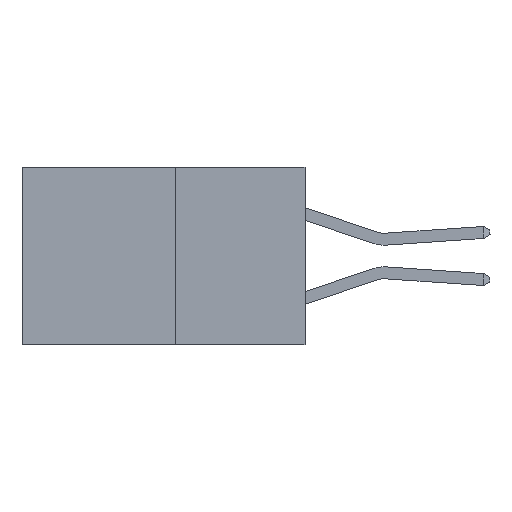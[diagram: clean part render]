
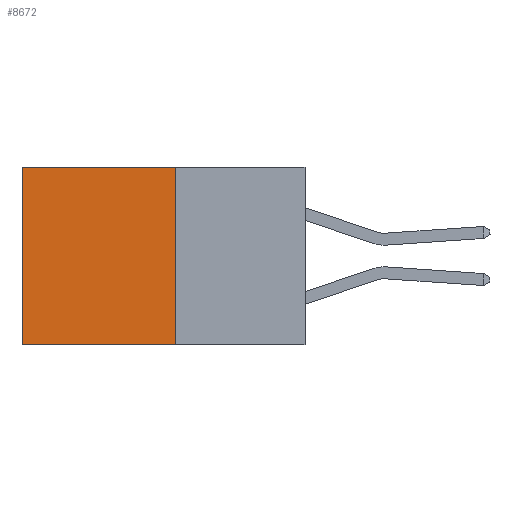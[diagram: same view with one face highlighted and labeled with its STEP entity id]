
A CAD part, left-side view. The second image highlights one B-rep face of the part: STEP entity #8672.
In plain terms, the highlighted planar face has unit normal (-1, 0, 0).
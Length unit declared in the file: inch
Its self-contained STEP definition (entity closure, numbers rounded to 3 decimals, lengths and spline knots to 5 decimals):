
#393 = EDGE_CURVE ( 'NONE', #8208, #5028, #4133, .T. ) ;
#781 = VECTOR ( 'NONE', #8328, 39.37008 ) ;
#1200 = VERTEX_POINT ( 'NONE', #11657 ) ;
#1939 = VERTEX_POINT ( 'NONE', #8195 ) ;
#2262 = CARTESIAN_POINT ( 'NONE',  ( 0.277, 0.59, -0.37 ) ) ;
#3747 = FACE_OUTER_BOUND ( 'NONE', #6007, .T. ) ;
#4133 = LINE ( 'NONE', #11971, #781 ) ;
#5028 = VERTEX_POINT ( 'NONE', #6715 ) ;
#5177 = EDGE_CURVE ( 'NONE', #1939, #1200, #8496, .T. ) ;
#5784 = VECTOR ( 'NONE', #11952, 39.37008 ) ;
#5949 = VECTOR ( 'NONE', #14698, 39.37008 ) ;
#6007 = EDGE_LOOP ( 'NONE', ( #10466, #9298, #6360, #11287 ) ) ;
#6179 = PLANE ( 'NONE',  #8177 ) ;
#6360 = ORIENTED_EDGE ( 'NONE', *, *, #15496, .F. ) ;
#6715 = CARTESIAN_POINT ( 'NONE',  ( 0.277, 0.59, 0. ) ) ;
#7384 = CARTESIAN_POINT ( 'NONE',  ( 0.277, 0.27, -0.37 ) ) ;
#8134 = VECTOR ( 'NONE', #11903, 39.37008 ) ;
#8177 = AXIS2_PLACEMENT_3D ( 'NONE', #7384, #15830, #8609 ) ;
#8195 = CARTESIAN_POINT ( 'NONE',  ( 0.277, 0.27, -0.37 ) ) ;
#8208 = VERTEX_POINT ( 'NONE', #11421 ) ;
#8328 = DIRECTION ( 'NONE',  ( 0., 1., 0. ) ) ;
#8496 = LINE ( 'NONE', #15437, #8134 ) ;
#8609 = DIRECTION ( 'NONE',  ( 0., 0., -1. ) ) ;
#8672 = ADVANCED_FACE ( 'NONE', ( #3747 ), #6179, .F. ) ;
#8994 = LINE ( 'NONE', #2262, #5784 ) ;
#9298 = ORIENTED_EDGE ( 'NONE', *, *, #5177, .F. ) ;
#10466 = ORIENTED_EDGE ( 'NONE', *, *, #15181, .T. ) ;
#11287 = ORIENTED_EDGE ( 'NONE', *, *, #393, .T. ) ;
#11421 = CARTESIAN_POINT ( 'NONE',  ( 0.277, 0.27, 0. ) ) ;
#11657 = CARTESIAN_POINT ( 'NONE',  ( 0.277, 0.59, -0.37 ) ) ;
#11903 = DIRECTION ( 'NONE',  ( 0., 1., 0. ) ) ;
#11952 = DIRECTION ( 'NONE',  ( 0., 0., -1. ) ) ;
#11971 = CARTESIAN_POINT ( 'NONE',  ( 0.277, 0.27, 0. ) ) ;
#12449 = LINE ( 'NONE', #13508, #5949 ) ;
#13508 = CARTESIAN_POINT ( 'NONE',  ( 0.277, 0.27, -0.37 ) ) ;
#14698 = DIRECTION ( 'NONE',  ( 0., 0., -1. ) ) ;
#15181 = EDGE_CURVE ( 'NONE', #5028, #1200, #8994, .T. ) ;
#15437 = CARTESIAN_POINT ( 'NONE',  ( 0.277, 0.27, -0.37 ) ) ;
#15496 = EDGE_CURVE ( 'NONE', #8208, #1939, #12449, .T. ) ;
#15830 = DIRECTION ( 'NONE',  ( 1., 0., 0. ) ) ;
